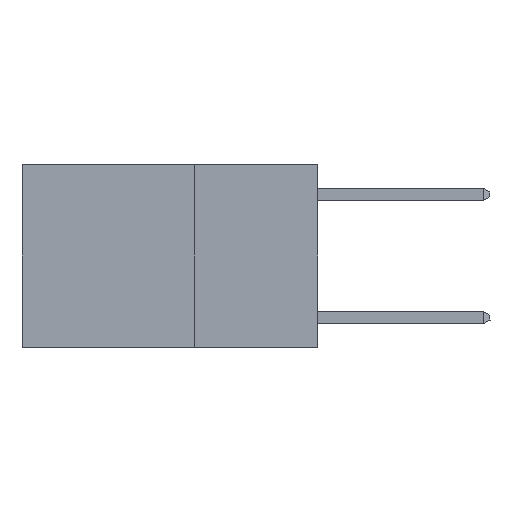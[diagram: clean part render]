
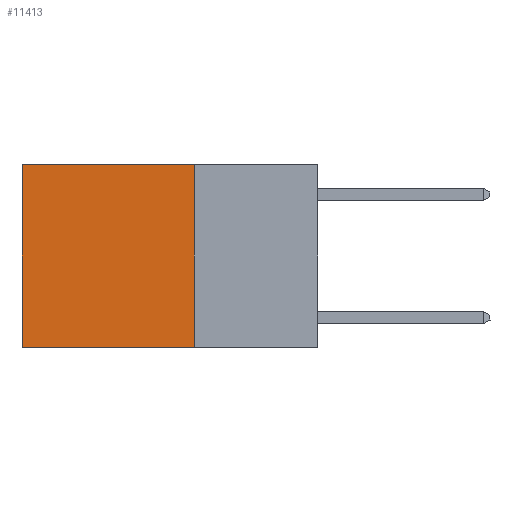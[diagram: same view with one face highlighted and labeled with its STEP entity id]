
A CAD part, left-side view. The second image highlights one B-rep face of the part: STEP entity #11413.
In plain terms, the highlighted planar face has unit normal (-1, 0, 0).
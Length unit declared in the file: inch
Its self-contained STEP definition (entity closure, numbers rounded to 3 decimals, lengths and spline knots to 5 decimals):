
#536 = EDGE_LOOP ( 'NONE', ( #6000, #10028, #9648, #6278 ) ) ;
#635 = EDGE_CURVE ( 'NONE', #7839, #1376, #2122, .T. ) ;
#1328 = VERTEX_POINT ( 'NONE', #6441 ) ;
#1376 = VERTEX_POINT ( 'NONE', #5861 ) ;
#2122 = LINE ( 'NONE', #10666, #6624 ) ;
#2776 = CARTESIAN_POINT ( 'NONE',  ( 0.2625, 0.25, -0.37 ) ) ;
#2945 = CARTESIAN_POINT ( 'NONE',  ( 0.2625, 0.6, 0. ) ) ;
#2971 = CARTESIAN_POINT ( 'NONE',  ( 0.2625, 0.25, 0. ) ) ;
#3392 = EDGE_CURVE ( 'NONE', #1328, #7839, #10899, .T. ) ;
#3652 = DIRECTION ( 'NONE',  ( 0., 0., -1. ) ) ;
#4612 = DIRECTION ( 'NONE',  ( 1., 0., 0. ) ) ;
#5723 = VERTEX_POINT ( 'NONE', #9637 ) ;
#5861 = CARTESIAN_POINT ( 'NONE',  ( 0.2625, 0.6, -0.37 ) ) ;
#6000 = ORIENTED_EDGE ( 'NONE', *, *, #8000, .T. ) ;
#6015 = VECTOR ( 'NONE', #3652, 39.37008 ) ;
#6031 = EDGE_CURVE ( 'NONE', #1328, #5723, #6240, .T. ) ;
#6240 = LINE ( 'NONE', #2971, #10849 ) ;
#6278 = ORIENTED_EDGE ( 'NONE', *, *, #6031, .T. ) ;
#6441 = CARTESIAN_POINT ( 'NONE',  ( 0.2625, 0.25, 0. ) ) ;
#6457 = DIRECTION ( 'NONE',  ( 0., 0., -1. ) ) ;
#6624 = VECTOR ( 'NONE', #10591, 39.37008 ) ;
#7055 = AXIS2_PLACEMENT_3D ( 'NONE', #9835, #4612, #10683 ) ;
#7241 = FACE_OUTER_BOUND ( 'NONE', #536, .T. ) ;
#7839 = VERTEX_POINT ( 'NONE', #2776 ) ;
#8000 = EDGE_CURVE ( 'NONE', #5723, #1376, #11095, .T. ) ;
#8119 = PLANE ( 'NONE',  #7055 ) ;
#9147 = DIRECTION ( 'NONE',  ( 0., 1., 0. ) ) ;
#9637 = CARTESIAN_POINT ( 'NONE',  ( 0.2625, 0.6, 0. ) ) ;
#9648 = ORIENTED_EDGE ( 'NONE', *, *, #3392, .F. ) ;
#9835 = CARTESIAN_POINT ( 'NONE',  ( 0.2625, 0.25, 0. ) ) ;
#10028 = ORIENTED_EDGE ( 'NONE', *, *, #635, .F. ) ;
#10591 = DIRECTION ( 'NONE',  ( 0., 1., 0. ) ) ;
#10620 = CARTESIAN_POINT ( 'NONE',  ( 0.2625, 0.25, 0. ) ) ;
#10666 = CARTESIAN_POINT ( 'NONE',  ( 0.2625, 0.25, -0.37 ) ) ;
#10683 = DIRECTION ( 'NONE',  ( 0., 0., -1. ) ) ;
#10826 = VECTOR ( 'NONE', #6457, 39.37008 ) ;
#10849 = VECTOR ( 'NONE', #9147, 39.37008 ) ;
#10899 = LINE ( 'NONE', #10620, #6015 ) ;
#11095 = LINE ( 'NONE', #2945, #10826 ) ;
#11413 = ADVANCED_FACE ( 'NONE', ( #7241 ), #8119, .F. ) ;
